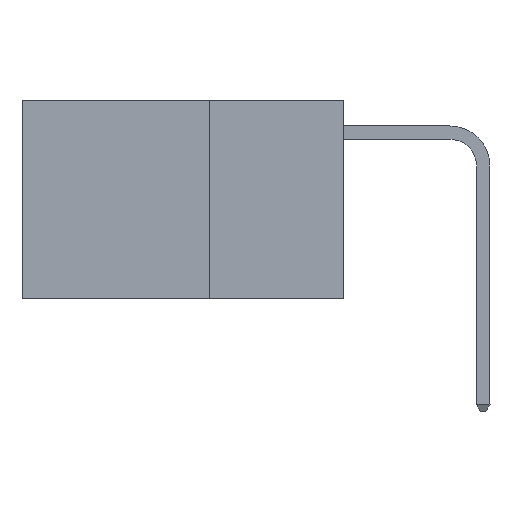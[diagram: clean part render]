
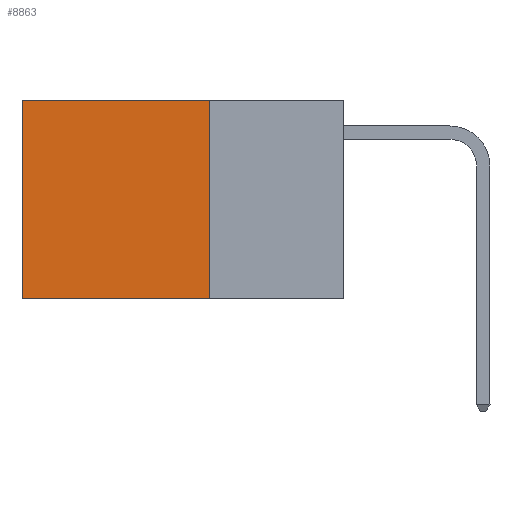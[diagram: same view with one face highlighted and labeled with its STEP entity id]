
A CAD part, left-side view. The second image highlights one B-rep face of the part: STEP entity #8863.
In plain terms, the highlighted planar face has unit normal (-1, 0, 0).
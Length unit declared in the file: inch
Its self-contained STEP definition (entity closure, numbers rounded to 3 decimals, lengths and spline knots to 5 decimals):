
#150 = EDGE_LOOP ( 'NONE', ( #2137, #915, #1360, #9030 ) ) ;
#224 = CARTESIAN_POINT ( 'NONE',  ( 0.2625, 0.6, -0.37 ) ) ;
#248 = CARTESIAN_POINT ( 'NONE',  ( 0.2625, 0.25, 0. ) ) ;
#564 = DIRECTION ( 'NONE',  ( 1., 0., 0. ) ) ;
#593 = EDGE_CURVE ( 'NONE', #2323, #2948, #11941, .T. ) ;
#637 = DIRECTION ( 'NONE',  ( 0., 0., -1. ) ) ;
#915 = ORIENTED_EDGE ( 'NONE', *, *, #11249, .F. ) ;
#916 = LINE ( 'NONE', #248, #11352 ) ;
#979 = CARTESIAN_POINT ( 'NONE',  ( 0.2625, 0.6, 0. ) ) ;
#1360 = ORIENTED_EDGE ( 'NONE', *, *, #2142, .F. ) ;
#1988 = CARTESIAN_POINT ( 'NONE',  ( 0.2625, 0.25, 0. ) ) ;
#2137 = ORIENTED_EDGE ( 'NONE', *, *, #593, .T. ) ;
#2142 = EDGE_CURVE ( 'NONE', #4045, #4803, #916, .T. ) ;
#2323 = VERTEX_POINT ( 'NONE', #6849 ) ;
#2601 = DIRECTION ( 'NONE',  ( 0., 1., 0. ) ) ;
#2688 = PLANE ( 'NONE',  #11518 ) ;
#2948 = VERTEX_POINT ( 'NONE', #224 ) ;
#3167 = DIRECTION ( 'NONE',  ( 0., 0., -1. ) ) ;
#3322 = CARTESIAN_POINT ( 'NONE',  ( 0.2625, 0.25, 0. ) ) ;
#3430 = EDGE_CURVE ( 'NONE', #4045, #2323, #11381, .T. ) ;
#3693 = CARTESIAN_POINT ( 'NONE',  ( 0.2625, 0.25, 0. ) ) ;
#4045 = VERTEX_POINT ( 'NONE', #3322 ) ;
#4803 = VERTEX_POINT ( 'NONE', #9918 ) ;
#6316 = VECTOR ( 'NONE', #6468, 39.37008 ) ;
#6468 = DIRECTION ( 'NONE',  ( 0., 1., 0. ) ) ;
#6849 = CARTESIAN_POINT ( 'NONE',  ( 0.2625, 0.6, 0. ) ) ;
#7938 = FACE_OUTER_BOUND ( 'NONE', #150, .T. ) ;
#8863 = ADVANCED_FACE ( 'NONE', ( #7938 ), #2688, .F. ) ;
#8888 = LINE ( 'NONE', #9949, #6316 ) ;
#9030 = ORIENTED_EDGE ( 'NONE', *, *, #3430, .T. ) ;
#9494 = VECTOR ( 'NONE', #9681, 39.37008 ) ;
#9681 = DIRECTION ( 'NONE',  ( 0., 0., -1. ) ) ;
#9918 = CARTESIAN_POINT ( 'NONE',  ( 0.2625, 0.25, -0.37 ) ) ;
#9949 = CARTESIAN_POINT ( 'NONE',  ( 0.2625, 0.25, -0.37 ) ) ;
#11249 = EDGE_CURVE ( 'NONE', #4803, #2948, #8888, .T. ) ;
#11352 = VECTOR ( 'NONE', #3167, 39.37008 ) ;
#11381 = LINE ( 'NONE', #3693, #11813 ) ;
#11518 = AXIS2_PLACEMENT_3D ( 'NONE', #1988, #564, #637 ) ;
#11813 = VECTOR ( 'NONE', #2601, 39.37008 ) ;
#11941 = LINE ( 'NONE', #979, #9494 ) ;
